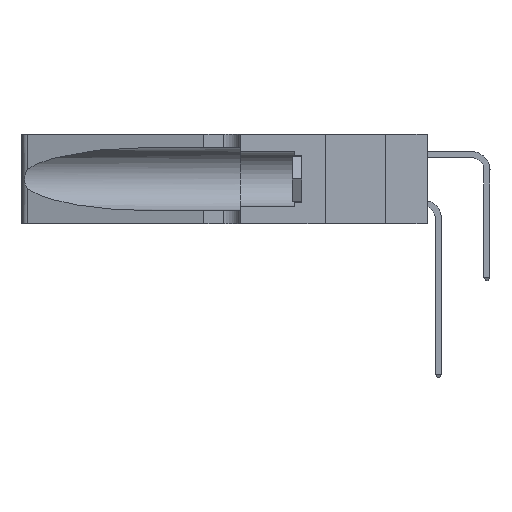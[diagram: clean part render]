
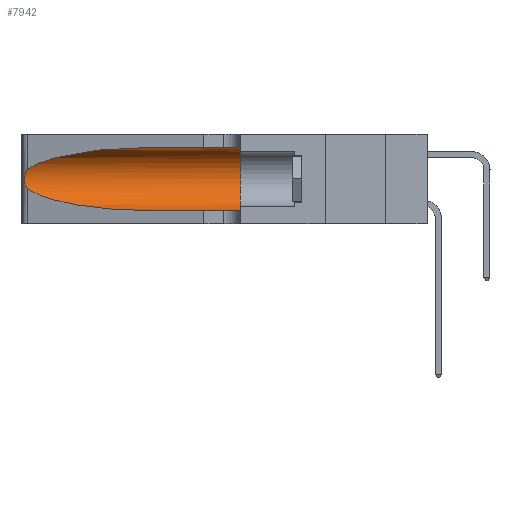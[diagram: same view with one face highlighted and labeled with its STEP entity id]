
A CAD part, left-side view. The second image highlights one B-rep face of the part: STEP entity #7942.
In plain terms, the highlighted cylindrical face has radius 3.308 mm (diameter 6.617 mm), a partial arc.
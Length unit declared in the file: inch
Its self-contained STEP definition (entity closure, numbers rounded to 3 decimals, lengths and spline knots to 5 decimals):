
#228 = CARTESIAN_POINT ( 'NONE',  ( 0.1305, 1.61858, 0.31525 ) ) ;
#902 = CARTESIAN_POINT ( 'NONE',  ( 0.25639, 1.23184, 0.21858 ) ) ;
#1053 = CARTESIAN_POINT ( 'NONE',  ( 0.26075, 1.23896, 0.19203 ) ) ;
#1229 = EDGE_CURVE ( 'NONE', #7481, #8401, #6077, .T. ) ;
#1316 = CARTESIAN_POINT ( 'NONE',  ( 0.2373, 1.15595, 0.28018 ) ) ;
#1565 = CARTESIAN_POINT ( 'NONE',  ( 0.1305, 0.35, 0.185 ) ) ;
#1806 =( BOUNDED_CURVE ( )  B_SPLINE_CURVE ( 3, ( #4710, #12064, #1316, #15668 ),
 .UNSPECIFIED., .F., .F. ) 
 B_SPLINE_CURVE_WITH_KNOTS ( ( 4, 4 ),
 ( 1.5708, 2.84003 ),
 .UNSPECIFIED. ) 
 CURVE ( )  GEOMETRIC_REPRESENTATION_ITEM ( )  RATIONAL_B_SPLINE_CURVE ( ( 1., 0.87, 0.87, 1. ) ) 
 REPRESENTATION_ITEM ( '' )  );
#2335 = CARTESIAN_POINT ( 'NONE',  ( 0.1305, 0.35, 0.05475 ) ) ;
#2999 = CARTESIAN_POINT ( 'NONE',  ( 0.26017, 1.23833, 0.17102 ) ) ;
#3379 = CARTESIAN_POINT ( 'NONE',  ( 0.1305, 0.72297, 0.05475 ) ) ;
#3464 = CARTESIAN_POINT ( 'NONE',  ( 0.25487, 1.22718, 0.14631 ) ) ;
#3544 = CARTESIAN_POINT ( 'NONE',  ( 0.18966, 0.96281, 0.05475 ) ) ;
#3828 = DIRECTION ( 'NONE',  ( 0., -1., 0. ) ) ;
#4550 = EDGE_LOOP ( 'NONE', ( #9695, #19033, #21287, #5386, #17012, #21345 ) ) ;
#4710 = CARTESIAN_POINT ( 'NONE',  ( 0.1305, 0.72297, 0.31525 ) ) ;
#4955 = DIRECTION ( 'NONE',  ( 0., 0., 1. ) ) ;
#5176 = VECTOR ( 'NONE', #3828, 39.37008 ) ;
#5386 = ORIENTED_EDGE ( 'NONE', *, *, #17489, .T. ) ;
#5615 = VECTOR ( 'NONE', #7517, 39.37008 ) ;
#5982 = EDGE_CURVE ( 'NONE', #7651, #10276, #10637, .T. ) ;
#6019 = CARTESIAN_POINT ( 'NONE',  ( 0.1305, 1.61858, 0.05475 ) ) ;
#6077 = LINE ( 'NONE', #228, #5176 ) ;
#6691 = CARTESIAN_POINT ( 'NONE',  ( 0.1305, 0.35, 0.31525 ) ) ;
#7016 = EDGE_CURVE ( 'NONE', #8556, #7651, #17269, .T. ) ;
#7024 = CARTESIAN_POINT ( 'NONE',  ( 0.25487, 1.22718, 0.14631 ) ) ;
#7049 = CARTESIAN_POINT ( 'NONE',  ( 0.1305, 1.61858, 0.185 ) ) ;
#7358 = EDGE_CURVE ( 'NONE', #8401, #14754, #19163, .T. ) ;
#7428 = AXIS2_PLACEMENT_3D ( 'NONE', #1565, #14199, #4955 ) ;
#7481 = VERTEX_POINT ( 'NONE', #21403 ) ;
#7517 = DIRECTION ( 'NONE',  ( 0., -1., 0. ) ) ;
#7651 = VERTEX_POINT ( 'NONE', #14272 ) ;
#7942 = ADVANCED_FACE ( 'NONE', ( #23186 ), #17044, .F. ) ;
#8161 = CARTESIAN_POINT ( 'NONE',  ( 0.25856, 1.23593, 0.16098 ) ) ;
#8333 = EDGE_CURVE ( 'NONE', #7481, #8556, #1806, .T. ) ;
#8401 = VERTEX_POINT ( 'NONE', #6691 ) ;
#8556 = VERTEX_POINT ( 'NONE', #14643 ) ;
#8881 = DIRECTION ( 'NONE',  ( 0., -1., 0. ) ) ;
#9695 = ORIENTED_EDGE ( 'NONE', *, *, #8333, .T. ) ;
#10212 = CARTESIAN_POINT ( 'NONE',  ( 0.25787, 1.23484, 0.2124 ) ) ;
#10276 = VERTEX_POINT ( 'NONE', #21930 ) ;
#10434 = CARTESIAN_POINT ( 'NONE',  ( 0.25555, 1.22993, 0.14849 ) ) ;
#10637 =( BOUNDED_CURVE ( )  B_SPLINE_CURVE ( 3, ( #3464, #12638, #3544, #3379 ),
 .UNSPECIFIED., .F., .F. ) 
 B_SPLINE_CURVE_WITH_KNOTS ( ( 4, 4 ),
 ( 3.44316, 4.71239 ),
 .UNSPECIFIED. ) 
 CURVE ( )  GEOMETRIC_REPRESENTATION_ITEM ( )  RATIONAL_B_SPLINE_CURVE ( ( 1., 0.87, 0.87, 1. ) ) 
 REPRESENTATION_ITEM ( '' )  );
#12064 = CARTESIAN_POINT ( 'NONE',  ( 0.18966, 0.96281, 0.31525 ) ) ;
#12638 = CARTESIAN_POINT ( 'NONE',  ( 0.2373, 1.15595, 0.08982 ) ) ;
#13755 = CARTESIAN_POINT ( 'NONE',  ( 0.25487, 1.22718, 0.22369 ) ) ;
#13821 = CARTESIAN_POINT ( 'NONE',  ( 0.25854, 1.2359, 0.20912 ) ) ;
#14199 = DIRECTION ( 'NONE',  ( 0., 1., 0. ) ) ;
#14272 = CARTESIAN_POINT ( 'NONE',  ( 0.25487, 1.22718, 0.14631 ) ) ;
#14643 = CARTESIAN_POINT ( 'NONE',  ( 0.25487, 1.22718, 0.22369 ) ) ;
#14754 = VERTEX_POINT ( 'NONE', #2335 ) ;
#15202 = LINE ( 'NONE', #6019, #5615 ) ;
#15394 = CARTESIAN_POINT ( 'NONE',  ( 0.25555, 1.22994, 0.2215 ) ) ;
#15621 = CARTESIAN_POINT ( 'NONE',  ( 0.26075, 1.23896, 0.178 ) ) ;
#15668 = CARTESIAN_POINT ( 'NONE',  ( 0.25487, 1.22718, 0.22369 ) ) ;
#17012 = ORIENTED_EDGE ( 'NONE', *, *, #7358, .F. ) ;
#17044 = CYLINDRICAL_SURFACE ( 'NONE', #22629, 0.13025 ) ;
#17269 = B_SPLINE_CURVE_WITH_KNOTS ( 'NONE', 3,
 ( #13755, #15394, #902, #10212, #13821, #19093, #1053, #15621, #2999, #8161, #22671, #22515, #10434, #7024 ),
 .UNSPECIFIED., .F., .F.,
 ( 4, 2, 2, 2, 2, 2, 4 ),
 ( 0., 0.00027, 0.00053, 0.00107, 0.0016, 0.00187, 0.00214 ),
 .UNSPECIFIED. ) ;
#17489 = EDGE_CURVE ( 'NONE', #10276, #14754, #15202, .T. ) ;
#19033 = ORIENTED_EDGE ( 'NONE', *, *, #7016, .T. ) ;
#19093 = CARTESIAN_POINT ( 'NONE',  ( 0.26018, 1.23835, 0.19895 ) ) ;
#19163 = CIRCLE ( 'NONE', #7428, 0.13025 ) ;
#21287 = ORIENTED_EDGE ( 'NONE', *, *, #5982, .T. ) ;
#21345 = ORIENTED_EDGE ( 'NONE', *, *, #1229, .F. ) ;
#21403 = CARTESIAN_POINT ( 'NONE',  ( 0.1305, 0.72297, 0.31525 ) ) ;
#21930 = CARTESIAN_POINT ( 'NONE',  ( 0.1305, 0.72297, 0.05475 ) ) ;
#22515 = CARTESIAN_POINT ( 'NONE',  ( 0.25639, 1.23186, 0.15144 ) ) ;
#22629 = AXIS2_PLACEMENT_3D ( 'NONE', #7049, #8881, #23217 ) ;
#22671 = CARTESIAN_POINT ( 'NONE',  ( 0.25789, 1.23486, 0.15765 ) ) ;
#23186 = FACE_OUTER_BOUND ( 'NONE', #4550, .T. ) ;
#23217 = DIRECTION ( 'NONE',  ( 0., 0., -1. ) ) ;
